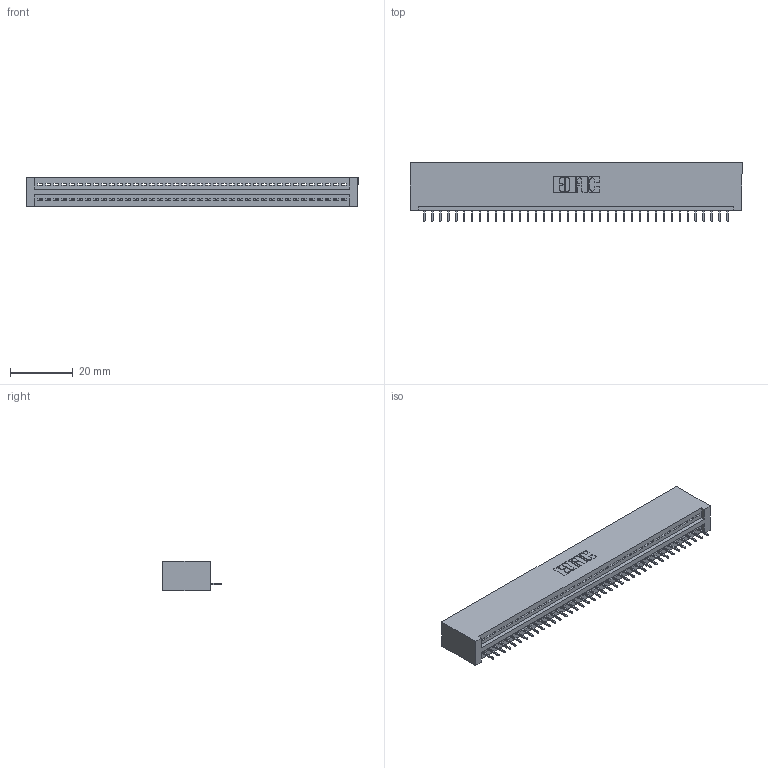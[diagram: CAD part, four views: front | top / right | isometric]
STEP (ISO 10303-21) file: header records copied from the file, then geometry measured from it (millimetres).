
FILE_DESCRIPTION (( 'STEP AP203' ), '1' );
FILE_NAME ('845-039-525-101.STEP', '2020-09-23T04:22:43', ( '' ), ( '' ), 'SwSTEP 2.0', 'SolidWorks 2020', '' );
FILE_SCHEMA (( 'CONFIG_CONTROL_DESIGN' ));
Length unit declared in the file: inch
Products named in the file (3): 345-292-001_345-293-125; 845 Part_No Mounting Lugs; 845-039-525-101
Assembly tree (40 placements, depth 2):
  845-039-525-101
    845 Part_No Mounting Lugs
    345-292-001_345-293-125  x39
Bounding box: 105.66 x 18.72 x 9.4 mm (x, y, z)
Volume: 10436.6 mm3; surface area: 13487.7 mm2
Topology: 40 solids, 40 shells, 2536 faces, 7337 edges, 4734 vertices
Faces by surface type: plane 1870, cylinder 666
Entity records: 29553 total; most frequent: CARTESIAN_POINT 5125, ORIENTED_EDGE 5098, DIRECTION 4475, EDGE_CURVE 2549, VECTOR 2273, LINE 2273, VERTEX_POINT 1694, AXIS2_PLACEMENT_3D 1101
